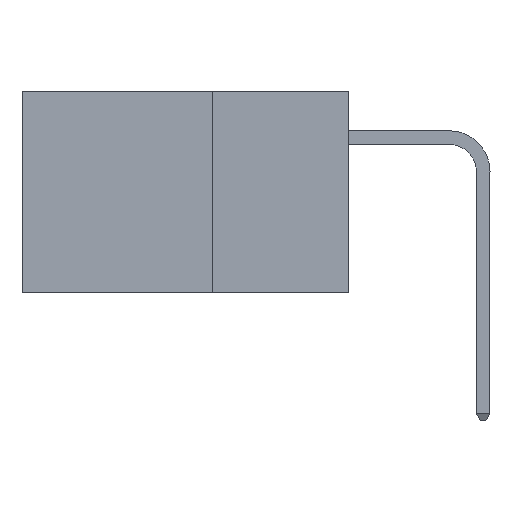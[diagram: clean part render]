
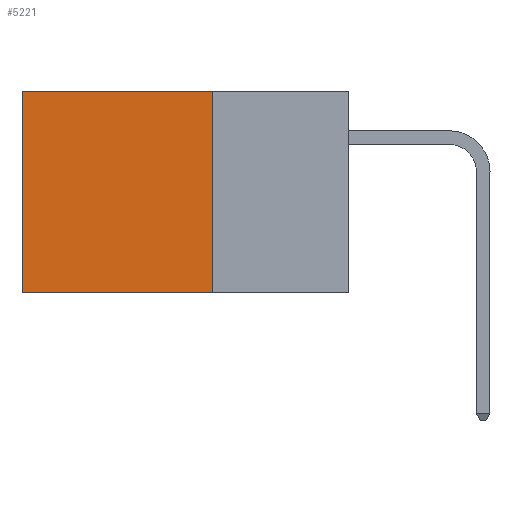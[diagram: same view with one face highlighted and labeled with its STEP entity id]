
A CAD part, left-side view. The second image highlights one B-rep face of the part: STEP entity #5221.
In plain terms, the highlighted planar face has unit normal (-1, 0, 0).
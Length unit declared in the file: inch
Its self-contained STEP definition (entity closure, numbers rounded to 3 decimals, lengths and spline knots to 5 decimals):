
#181 = VECTOR ( 'NONE', #6432, 39.37008 ) ;
#318 = EDGE_CURVE ( 'NONE', #8696, #3270, #1437, .T. ) ;
#598 = VECTOR ( 'NONE', #3353, 39.37008 ) ;
#611 = LINE ( 'NONE', #7477, #598 ) ;
#753 = LINE ( 'NONE', #5920, #6713 ) ;
#906 = DIRECTION ( 'NONE',  ( 0., 0., -1. ) ) ;
#1057 = VERTEX_POINT ( 'NONE', #4825 ) ;
#1437 = LINE ( 'NONE', #4671, #181 ) ;
#1441 = CARTESIAN_POINT ( 'NONE',  ( 0.2875, 0.6, 0. ) ) ;
#1472 = CARTESIAN_POINT ( 'NONE',  ( 0.2875, 0.25, 0. ) ) ;
#2035 = EDGE_CURVE ( 'NONE', #8696, #1057, #2589, .T. ) ;
#2067 = ORIENTED_EDGE ( 'NONE', *, *, #318, .T. ) ;
#2390 = DIRECTION ( 'NONE',  ( 0., 1., 0. ) ) ;
#2589 = LINE ( 'NONE', #6021, #11034 ) ;
#2728 = ORIENTED_EDGE ( 'NONE', *, *, #5737, .T. ) ;
#3270 = VERTEX_POINT ( 'NONE', #1441 ) ;
#3353 = DIRECTION ( 'NONE',  ( 0., 0., -1. ) ) ;
#4496 = VERTEX_POINT ( 'NONE', #7609 ) ;
#4671 = CARTESIAN_POINT ( 'NONE',  ( 0.2875, 0.25, 0. ) ) ;
#4825 = CARTESIAN_POINT ( 'NONE',  ( 0.2875, 0.25, -0.37 ) ) ;
#4880 = FACE_OUTER_BOUND ( 'NONE', #5264, .T. ) ;
#5101 = DIRECTION ( 'NONE',  ( 0., 0., -1. ) ) ;
#5221 = ADVANCED_FACE ( 'NONE', ( #4880 ), #6008, .F. ) ;
#5264 = EDGE_LOOP ( 'NONE', ( #2728, #6621, #5526, #2067 ) ) ;
#5526 = ORIENTED_EDGE ( 'NONE', *, *, #2035, .F. ) ;
#5737 = EDGE_CURVE ( 'NONE', #3270, #4496, #611, .T. ) ;
#5811 = CARTESIAN_POINT ( 'NONE',  ( 0.2875, 0.25, 0. ) ) ;
#5920 = CARTESIAN_POINT ( 'NONE',  ( 0.2875, 0.25, -0.37 ) ) ;
#6008 = PLANE ( 'NONE',  #8501 ) ;
#6021 = CARTESIAN_POINT ( 'NONE',  ( 0.2875, 0.25, 0. ) ) ;
#6432 = DIRECTION ( 'NONE',  ( 0., 1., 0. ) ) ;
#6621 = ORIENTED_EDGE ( 'NONE', *, *, #7386, .F. ) ;
#6713 = VECTOR ( 'NONE', #2390, 39.37008 ) ;
#7386 = EDGE_CURVE ( 'NONE', #1057, #4496, #753, .T. ) ;
#7477 = CARTESIAN_POINT ( 'NONE',  ( 0.2875, 0.6, 0. ) ) ;
#7609 = CARTESIAN_POINT ( 'NONE',  ( 0.2875, 0.6, -0.37 ) ) ;
#8501 = AXIS2_PLACEMENT_3D ( 'NONE', #1472, #9284, #5101 ) ;
#8696 = VERTEX_POINT ( 'NONE', #5811 ) ;
#9284 = DIRECTION ( 'NONE',  ( 1., 0., 0. ) ) ;
#11034 = VECTOR ( 'NONE', #906, 39.37008 ) ;
